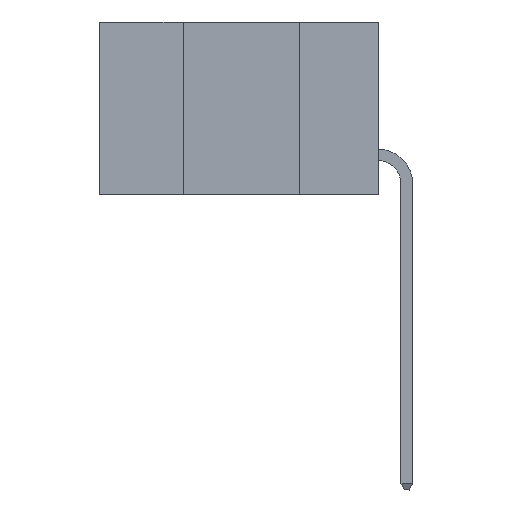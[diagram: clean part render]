
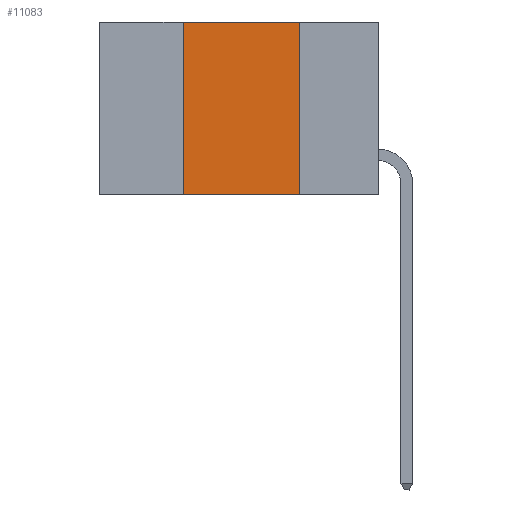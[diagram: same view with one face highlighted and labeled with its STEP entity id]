
A CAD part, left-side view. The second image highlights one B-rep face of the part: STEP entity #11083.
In plain terms, the highlighted planar face has unit normal (-1, 0, 0).
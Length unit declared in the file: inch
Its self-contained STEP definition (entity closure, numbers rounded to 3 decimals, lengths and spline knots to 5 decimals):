
#649 = EDGE_CURVE ( 'NONE', #11066, #15370, #2052, .T. ) ;
#2052 = LINE ( 'NONE', #12493, #6435 ) ;
#2511 = LINE ( 'NONE', #13942, #7046 ) ;
#2944 = VECTOR ( 'NONE', #10900, 39.37008 ) ;
#3981 = LINE ( 'NONE', #11726, #7387 ) ;
#4100 = CARTESIAN_POINT ( 'NONE',  ( 0., 0.6, 0. ) ) ;
#4347 = CARTESIAN_POINT ( 'NONE',  ( 0., 0.42, -0.37 ) ) ;
#4563 = CARTESIAN_POINT ( 'NONE',  ( 0., 0.17, 0. ) ) ;
#5545 = CARTESIAN_POINT ( 'NONE',  ( 0., 0.17, -0.37 ) ) ;
#5941 = VERTEX_POINT ( 'NONE', #4563 ) ;
#6065 = DIRECTION ( 'NONE',  ( 0., 0., -1. ) ) ;
#6435 = VECTOR ( 'NONE', #7141, 39.37008 ) ;
#6578 = EDGE_CURVE ( 'NONE', #5941, #15370, #3981, .T. ) ;
#6882 = ORIENTED_EDGE ( 'NONE', *, *, #14411, .F. ) ;
#7046 = VECTOR ( 'NONE', #15194, 39.37008 ) ;
#7052 = CARTESIAN_POINT ( 'NONE',  ( 0., 0.42, -0.37 ) ) ;
#7141 = DIRECTION ( 'NONE',  ( 0., -1., 0. ) ) ;
#7387 = VECTOR ( 'NONE', #10563, 39.37008 ) ;
#9186 = DIRECTION ( 'NONE',  ( 1., 0., 0. ) ) ;
#9877 = EDGE_CURVE ( 'NONE', #11066, #13701, #9901, .T. ) ;
#9901 = LINE ( 'NONE', #7052, #2944 ) ;
#10563 = DIRECTION ( 'NONE',  ( 0., 0., -1. ) ) ;
#10835 = FACE_OUTER_BOUND ( 'NONE', #14795, .T. ) ;
#10900 = DIRECTION ( 'NONE',  ( 0., 0., 1. ) ) ;
#11066 = VERTEX_POINT ( 'NONE', #4347 ) ;
#11083 = ADVANCED_FACE ( 'NONE', ( #10835 ), #11929, .F. ) ;
#11235 = AXIS2_PLACEMENT_3D ( 'NONE', #4100, #9186, #6065 ) ;
#11549 = ORIENTED_EDGE ( 'NONE', *, *, #6578, .F. ) ;
#11726 = CARTESIAN_POINT ( 'NONE',  ( 0., 0.17, -0.37 ) ) ;
#11929 = PLANE ( 'NONE',  #11235 ) ;
#12474 = ORIENTED_EDGE ( 'NONE', *, *, #9877, .F. ) ;
#12493 = CARTESIAN_POINT ( 'NONE',  ( 0., 0.6, -0.37 ) ) ;
#12766 = ORIENTED_EDGE ( 'NONE', *, *, #649, .T. ) ;
#13701 = VERTEX_POINT ( 'NONE', #14403 ) ;
#13942 = CARTESIAN_POINT ( 'NONE',  ( 0., 0.6, 0. ) ) ;
#14403 = CARTESIAN_POINT ( 'NONE',  ( 0., 0.42, 0. ) ) ;
#14411 = EDGE_CURVE ( 'NONE', #13701, #5941, #2511, .T. ) ;
#14795 = EDGE_LOOP ( 'NONE', ( #11549, #6882, #12474, #12766 ) ) ;
#15194 = DIRECTION ( 'NONE',  ( 0., -1., 0. ) ) ;
#15370 = VERTEX_POINT ( 'NONE', #5545 ) ;
